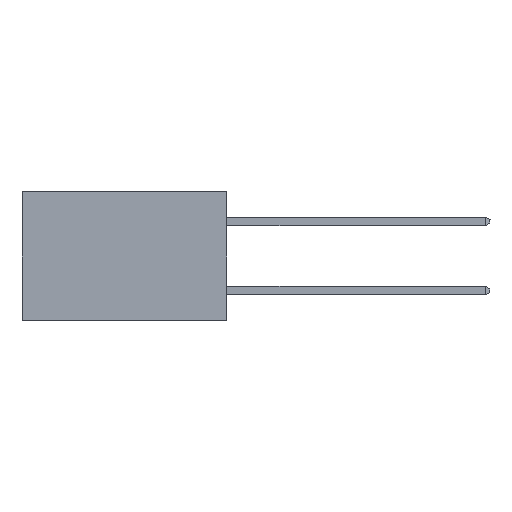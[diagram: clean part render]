
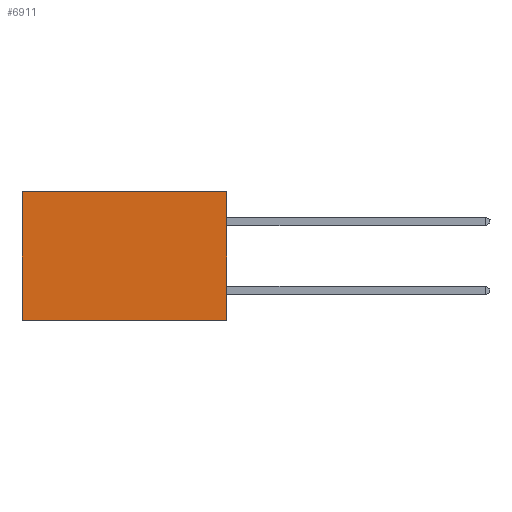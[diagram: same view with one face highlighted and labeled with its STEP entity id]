
A CAD part, left-side view. The second image highlights one B-rep face of the part: STEP entity #6911.
In plain terms, the highlighted planar face has unit normal (-1, 0, 0).
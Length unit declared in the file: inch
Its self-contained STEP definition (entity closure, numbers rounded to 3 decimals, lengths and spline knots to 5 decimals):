
#51 = EDGE_CURVE ( 'NONE', #18082, #27811, #21040, .T. ) ;
#130 = LINE ( 'NONE', #9769, #19872 ) ;
#662 = ORIENTED_EDGE ( 'NONE', *, *, #14412, .T. ) ;
#1723 = VECTOR ( 'NONE', #23668, 39.37008 ) ;
#3153 = ORIENTED_EDGE ( 'NONE', *, *, #19879, .T. ) ;
#3542 = VECTOR ( 'NONE', #12601, 39.37008 ) ;
#6911 = ADVANCED_FACE ( 'NONE', ( #26967 ), #17232, .F. ) ;
#7893 = DIRECTION ( 'NONE',  ( 0., 0., -1. ) ) ;
#8259 = CARTESIAN_POINT ( 'NONE',  ( 0.277, 0.59, -0.37 ) ) ;
#9569 = ORIENTED_EDGE ( 'NONE', *, *, #29517, .F. ) ;
#9769 = CARTESIAN_POINT ( 'NONE',  ( 0.277, 0., 0. ) ) ;
#12037 = DIRECTION ( 'NONE',  ( 0., 0., -1. ) ) ;
#12258 = DIRECTION ( 'NONE',  ( 1., 0., 0. ) ) ;
#12298 = CARTESIAN_POINT ( 'NONE',  ( 0.277, 0., -0.37 ) ) ;
#12302 = CARTESIAN_POINT ( 'NONE',  ( 0.277, 0., -0.37 ) ) ;
#12601 = DIRECTION ( 'NONE',  ( 0., 1., 0. ) ) ;
#12703 = VECTOR ( 'NONE', #7893, 39.37008 ) ;
#14412 = EDGE_CURVE ( 'NONE', #28823, #19886, #130, .T. ) ;
#15957 = EDGE_LOOP ( 'NONE', ( #3153, #22025, #9569, #662 ) ) ;
#17232 = PLANE ( 'NONE',  #28949 ) ;
#18082 = VERTEX_POINT ( 'NONE', #23169 ) ;
#19872 = VECTOR ( 'NONE', #24101, 39.37008 ) ;
#19879 = EDGE_CURVE ( 'NONE', #19886, #27811, #23880, .T. ) ;
#19886 = VERTEX_POINT ( 'NONE', #24505 ) ;
#21040 = LINE ( 'NONE', #12302, #3542 ) ;
#22025 = ORIENTED_EDGE ( 'NONE', *, *, #51, .F. ) ;
#22130 = CARTESIAN_POINT ( 'NONE',  ( 0.277, 0.59, -0.37 ) ) ;
#23169 = CARTESIAN_POINT ( 'NONE',  ( 0.277, 0., -0.37 ) ) ;
#23668 = DIRECTION ( 'NONE',  ( 0., 0., -1. ) ) ;
#23769 = CARTESIAN_POINT ( 'NONE',  ( 0.277, 0., -0.37 ) ) ;
#23880 = LINE ( 'NONE', #22130, #12703 ) ;
#24101 = DIRECTION ( 'NONE',  ( 0., 1., 0. ) ) ;
#24505 = CARTESIAN_POINT ( 'NONE',  ( 0.277, 0.59, 0. ) ) ;
#26934 = LINE ( 'NONE', #23769, #1723 ) ;
#26967 = FACE_OUTER_BOUND ( 'NONE', #15957, .T. ) ;
#27811 = VERTEX_POINT ( 'NONE', #8259 ) ;
#28026 = CARTESIAN_POINT ( 'NONE',  ( 0.277, 0., 0. ) ) ;
#28823 = VERTEX_POINT ( 'NONE', #28026 ) ;
#28949 = AXIS2_PLACEMENT_3D ( 'NONE', #12298, #12258, #12037 ) ;
#29517 = EDGE_CURVE ( 'NONE', #28823, #18082, #26934, .T. ) ;
